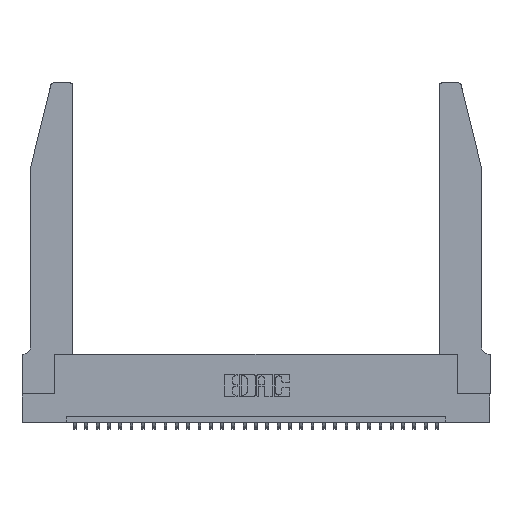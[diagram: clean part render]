
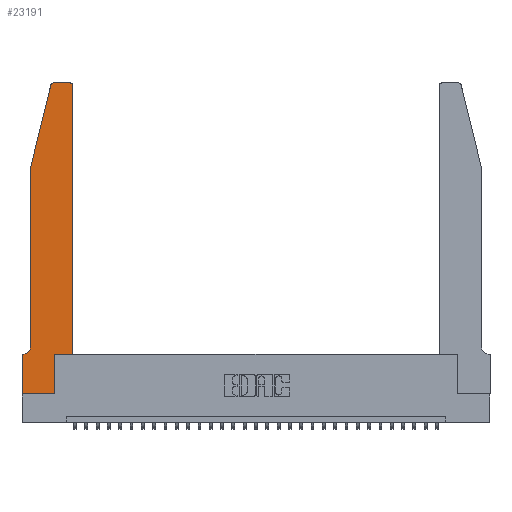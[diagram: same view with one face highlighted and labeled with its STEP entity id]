
A CAD part, top view. The second image highlights one B-rep face of the part: STEP entity #23191.
In plain terms, the highlighted planar face has unit normal (0, 0, 1).
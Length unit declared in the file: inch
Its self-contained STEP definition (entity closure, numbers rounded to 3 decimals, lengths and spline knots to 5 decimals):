
#36 = VECTOR ( 'NONE', #30101, 39.37008 ) ;
#131 = EDGE_CURVE ( 'NONE', #22185, #24532, #26204, .T. ) ;
#157 = AXIS2_PLACEMENT_3D ( 'NONE', #6267, #27779, #13437 ) ;
#387 = VECTOR ( 'NONE', #14403, 39.37008 ) ;
#485 = ORIENTED_EDGE ( 'NONE', *, *, #23079, .T. ) ;
#911 = LINE ( 'NONE', #14008, #4684 ) ;
#931 = CARTESIAN_POINT ( 'NONE',  ( 0.4205, 2.72, 0.37 ) ) ;
#1022 = CARTESIAN_POINT ( 'NONE',  ( 0., 0., 0.37 ) ) ;
#1231 = ORIENTED_EDGE ( 'NONE', *, *, #22566, .T. ) ;
#1305 = VERTEX_POINT ( 'NONE', #21119 ) ;
#1454 = CARTESIAN_POINT ( 'NONE',  ( 0.0755, 0.35, 0.37 ) ) ;
#2035 = EDGE_CURVE ( 'NONE', #19000, #27752, #15958, .T. ) ;
#2054 = VECTOR ( 'NONE', #21218, 39.37008 ) ;
#2234 = CARTESIAN_POINT ( 'NONE',  ( 0., 0.35, 0.37 ) ) ;
#2280 = CARTESIAN_POINT ( 'NONE',  ( 0.284, 2.72, 0.37 ) ) ;
#3114 = ORIENTED_EDGE ( 'NONE', *, *, #30853, .T. ) ;
#4211 = AXIS2_PLACEMENT_3D ( 'NONE', #931, #27522, #22483 ) ;
#4221 = CIRCLE ( 'NONE', #157, 0.07 ) ;
#4280 = CARTESIAN_POINT ( 'NONE',  ( 0.0755, 2., 0.37 ) ) ;
#4323 = CARTESIAN_POINT ( 'NONE',  ( 0.25487, 2.72718, 0.37 ) ) ;
#4419 = ORIENTED_EDGE ( 'NONE', *, *, #2035, .T. ) ;
#4469 = VERTEX_POINT ( 'NONE', #20457 ) ;
#4562 = AXIS2_PLACEMENT_3D ( 'NONE', #2280, #21296, #28227 ) ;
#4684 = VECTOR ( 'NONE', #4797, 39.37008 ) ;
#4797 = DIRECTION ( 'NONE',  ( 0., 1., 0. ) ) ;
#4961 = FACE_OUTER_BOUND ( 'NONE', #24086, .T. ) ;
#5574 = VECTOR ( 'NONE', #15866, 39.37008 ) ;
#6267 = CARTESIAN_POINT ( 'NONE',  ( 0.0055, 0.42, 0.37 ) ) ;
#6810 = VECTOR ( 'NONE', #12860, 39.37008 ) ;
#7178 = DIRECTION ( 'NONE',  ( 0., 0., 1. ) ) ;
#7464 = EDGE_CURVE ( 'NONE', #27752, #24427, #8988, .T. ) ;
#7468 = VERTEX_POINT ( 'NONE', #13913 ) ;
#7469 = ORIENTED_EDGE ( 'NONE', *, *, #10243, .T. ) ;
#7477 = LINE ( 'NONE', #9035, #36 ) ;
#8344 = LINE ( 'NONE', #14308, #2054 ) ;
#8621 = CARTESIAN_POINT ( 'NONE',  ( 0.2605, 2.75, 0.37 ) ) ;
#8988 = LINE ( 'NONE', #4280, #9675 ) ;
#9035 = CARTESIAN_POINT ( 'NONE',  ( 0.4505, 0.35, 0.37 ) ) ;
#9074 = VERTEX_POINT ( 'NONE', #18787 ) ;
#9409 = VERTEX_POINT ( 'NONE', #1022 ) ;
#9507 = ORIENTED_EDGE ( 'NONE', *, *, #13979, .T. ) ;
#9675 = VECTOR ( 'NONE', #23327, 39.37008 ) ;
#9885 = VECTOR ( 'NONE', #11976, 39.37008 ) ;
#10243 = EDGE_CURVE ( 'NONE', #4469, #1305, #15433, .T. ) ;
#10412 = LINE ( 'NONE', #1454, #5574 ) ;
#11135 = ORIENTED_EDGE ( 'NONE', *, *, #11839, .T. ) ;
#11839 = EDGE_CURVE ( 'NONE', #13606, #22185, #17622, .T. ) ;
#11946 = PLANE ( 'NONE',  #13327 ) ;
#11970 = CARTESIAN_POINT ( 'NONE',  ( 0.284, 2.75, 0.37 ) ) ;
#11976 = DIRECTION ( 'NONE',  ( 0., 1., 0. ) ) ;
#12860 = DIRECTION ( 'NONE',  ( -1., 0., 0. ) ) ;
#13327 = AXIS2_PLACEMENT_3D ( 'NONE', #2234, #7178, #16635 ) ;
#13437 = DIRECTION ( 'NONE',  ( -1., 0., 0. ) ) ;
#13546 = ORIENTED_EDGE ( 'NONE', *, *, #18631, .T. ) ;
#13606 = VERTEX_POINT ( 'NONE', #17946 ) ;
#13913 = CARTESIAN_POINT ( 'NONE',  ( 0., 0.35, 0.37 ) ) ;
#13979 = EDGE_CURVE ( 'NONE', #1305, #22859, #7477, .T. ) ;
#14008 = CARTESIAN_POINT ( 'NONE',  ( 0.4505, 0.35, 0.37 ) ) ;
#14288 = EDGE_CURVE ( 'NONE', #9409, #4469, #23156, .T. ) ;
#14308 = CARTESIAN_POINT ( 'NONE',  ( 0., 0., 0.37 ) ) ;
#14403 = DIRECTION ( 'NONE',  ( 1., 0., 0. ) ) ;
#15433 = LINE ( 'NONE', #28217, #9885 ) ;
#15866 = DIRECTION ( 'NONE',  ( -1., 0., 0. ) ) ;
#15958 = LINE ( 'NONE', #27489, #23832 ) ;
#16635 = DIRECTION ( 'NONE',  ( 1., 0., 0. ) ) ;
#17288 = CARTESIAN_POINT ( 'NONE',  ( 0.4505, 0.35, 0.37 ) ) ;
#17622 = CIRCLE ( 'NONE', #4211, 0.03 ) ;
#17946 = CARTESIAN_POINT ( 'NONE',  ( 0.4505, 2.72, 0.37 ) ) ;
#18631 = EDGE_CURVE ( 'NONE', #9074, #7468, #10412, .T. ) ;
#18787 = CARTESIAN_POINT ( 'NONE',  ( 0.0055, 0.35, 0.37 ) ) ;
#19000 = VERTEX_POINT ( 'NONE', #4323 ) ;
#19262 = ORIENTED_EDGE ( 'NONE', *, *, #30737, .T. ) ;
#20162 = DIRECTION ( 'NONE',  ( -0.239, -0.971, 0. ) ) ;
#20457 = CARTESIAN_POINT ( 'NONE',  ( 0.2865, 0., 0.37 ) ) ;
#21119 = CARTESIAN_POINT ( 'NONE',  ( 0.2865, 0.35, 0.37 ) ) ;
#21218 = DIRECTION ( 'NONE',  ( 0., -1., 0. ) ) ;
#21296 = DIRECTION ( 'NONE',  ( 0., 0., 1. ) ) ;
#21361 = ORIENTED_EDGE ( 'NONE', *, *, #7464, .T. ) ;
#21528 = CARTESIAN_POINT ( 'NONE',  ( 0., 0., 0.37 ) ) ;
#22185 = VERTEX_POINT ( 'NONE', #24263 ) ;
#22483 = DIRECTION ( 'NONE',  ( 1., 0., 0. ) ) ;
#22566 = EDGE_CURVE ( 'NONE', #24532, #19000, #30703, .T. ) ;
#22596 = ORIENTED_EDGE ( 'NONE', *, *, #131, .T. ) ;
#22859 = VERTEX_POINT ( 'NONE', #17288 ) ;
#23079 = EDGE_CURVE ( 'NONE', #24427, #9074, #4221, .T. ) ;
#23156 = LINE ( 'NONE', #21528, #387 ) ;
#23191 = ADVANCED_FACE ( 'NONE', ( #4961 ), #11946, .T. ) ;
#23327 = DIRECTION ( 'NONE',  ( 0., -1., 0. ) ) ;
#23832 = VECTOR ( 'NONE', #20162, 39.37008 ) ;
#24086 = EDGE_LOOP ( 'NONE', ( #22596, #1231, #4419, #21361, #485, #13546, #19262, #25206, #7469, #9507, #3114, #11135 ) ) ;
#24263 = CARTESIAN_POINT ( 'NONE',  ( 0.4205, 2.75, 0.37 ) ) ;
#24427 = VERTEX_POINT ( 'NONE', #30690 ) ;
#24532 = VERTEX_POINT ( 'NONE', #11970 ) ;
#25206 = ORIENTED_EDGE ( 'NONE', *, *, #14288, .T. ) ;
#26204 = LINE ( 'NONE', #8621, #6810 ) ;
#27489 = CARTESIAN_POINT ( 'NONE',  ( 0.0755, 2., 0.37 ) ) ;
#27522 = DIRECTION ( 'NONE',  ( 0., 0., 1. ) ) ;
#27752 = VERTEX_POINT ( 'NONE', #28325 ) ;
#27779 = DIRECTION ( 'NONE',  ( 0., 0., -1. ) ) ;
#28217 = CARTESIAN_POINT ( 'NONE',  ( 0.2865, 0.35, 0.37 ) ) ;
#28227 = DIRECTION ( 'NONE',  ( 1., 0., 0. ) ) ;
#28325 = CARTESIAN_POINT ( 'NONE',  ( 0.0755, 2., 0.37 ) ) ;
#30101 = DIRECTION ( 'NONE',  ( 1., 0., 0. ) ) ;
#30690 = CARTESIAN_POINT ( 'NONE',  ( 0.0755, 0.42, 0.37 ) ) ;
#30703 = CIRCLE ( 'NONE', #4562, 0.03 ) ;
#30737 = EDGE_CURVE ( 'NONE', #7468, #9409, #8344, .T. ) ;
#30853 = EDGE_CURVE ( 'NONE', #22859, #13606, #911, .T. ) ;
